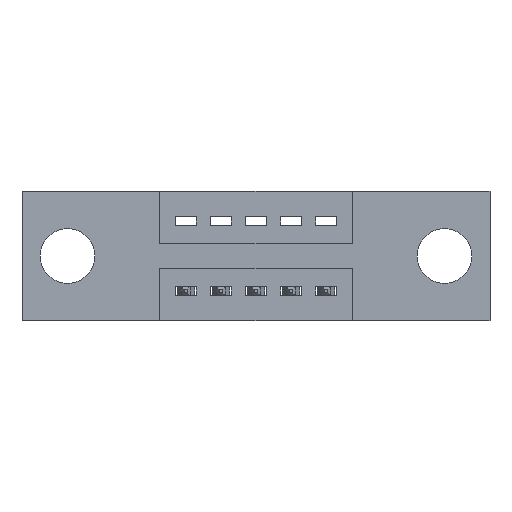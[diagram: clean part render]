
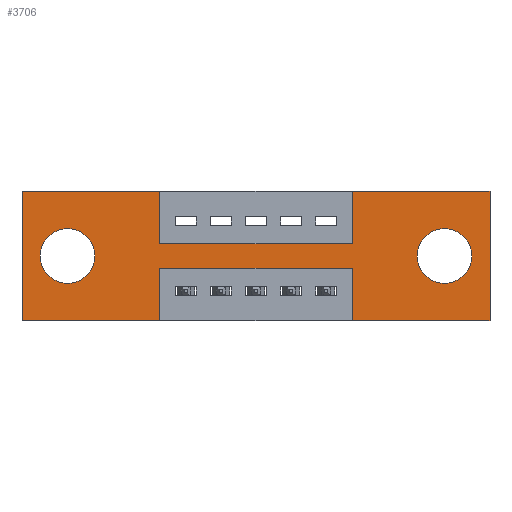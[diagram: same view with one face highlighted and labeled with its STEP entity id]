
A CAD part, front view. The second image highlights one B-rep face of the part: STEP entity #3706.
In plain terms, the highlighted planar face has unit normal (0, -1, 0).
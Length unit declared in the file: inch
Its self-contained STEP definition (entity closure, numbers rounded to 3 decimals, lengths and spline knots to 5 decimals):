
#21 = VERTEX_POINT ( 'NONE', #4066 ) ;
#74 = ORIENTED_EDGE ( 'NONE', *, *, #4020, .T. ) ;
#341 = CIRCLE ( 'NONE', #486, 0.078 ) ;
#416 = VERTEX_POINT ( 'NONE', #6061 ) ;
#418 = FACE_BOUND ( 'NONE', #1956, .T. ) ;
#486 = AXIS2_PLACEMENT_3D ( 'NONE', #2721, #8781, #7481 ) ;
#595 = AXIS2_PLACEMENT_3D ( 'NONE', #3343, #1869, #6625 ) ;
#641 = DIRECTION ( 'NONE',  ( 0., 1., 0. ) ) ;
#747 = AXIS2_PLACEMENT_3D ( 'NONE', #6677, #6643, #4599 ) ;
#905 = CARTESIAN_POINT ( 'NONE',  ( 0.9425, 0., -0.37 ) ) ;
#945 = VECTOR ( 'NONE', #3527, 39.37008 ) ;
#966 = VECTOR ( 'NONE', #6307, 39.37008 ) ;
#1000 = DIRECTION ( 'NONE',  ( 0., 0., 1. ) ) ;
#1029 = EDGE_CURVE ( 'NONE', #7774, #8764, #7888, .T. ) ;
#1031 = DIRECTION ( 'NONE',  ( 0., 0., -1. ) ) ;
#1033 = DIRECTION ( 'NONE',  ( -1., 0., 0. ) ) ;
#1087 = CARTESIAN_POINT ( 'NONE',  ( 1.335, 0., 0. ) ) ;
#1292 = LINE ( 'NONE', #8317, #966 ) ;
#1485 = EDGE_CURVE ( 'NONE', #3220, #4283, #3207, .T. ) ;
#1566 = CIRCLE ( 'NONE', #7570, 0.078 ) ;
#1573 = CARTESIAN_POINT ( 'NONE',  ( 1.205, 0., -0.107 ) ) ;
#1627 = ORIENTED_EDGE ( 'NONE', *, *, #7417, .T. ) ;
#1657 = CARTESIAN_POINT ( 'NONE',  ( 0.3925, 0., -0.15 ) ) ;
#1842 = DIRECTION ( 'NONE',  ( 1., 0., 0. ) ) ;
#1860 = ORIENTED_EDGE ( 'NONE', *, *, #8608, .F. ) ;
#1869 = DIRECTION ( 'NONE',  ( 0., -1., 0. ) ) ;
#1956 = EDGE_LOOP ( 'NONE', ( #74, #4392 ) ) ;
#2031 = CARTESIAN_POINT ( 'NONE',  ( 1.335, 0., 0. ) ) ;
#2058 = VERTEX_POINT ( 'NONE', #1657 ) ;
#2190 = LINE ( 'NONE', #3152, #5684 ) ;
#2250 = CARTESIAN_POINT ( 'NONE',  ( 0.3925, 0., -0.22 ) ) ;
#2300 = EDGE_CURVE ( 'NONE', #8406, #6482, #341, .T. ) ;
#2382 = VERTEX_POINT ( 'NONE', #8207 ) ;
#2653 = ORIENTED_EDGE ( 'NONE', *, *, #7358, .F. ) ;
#2720 = VERTEX_POINT ( 'NONE', #4637 ) ;
#2721 = CARTESIAN_POINT ( 'NONE',  ( 0.13, 0., -0.185 ) ) ;
#2741 = LINE ( 'NONE', #2250, #7955 ) ;
#2833 = EDGE_CURVE ( 'NONE', #6763, #5205, #5071, .T. ) ;
#2945 = ORIENTED_EDGE ( 'NONE', *, *, #3050, .F. ) ;
#3024 = VECTOR ( 'NONE', #6362, 39.37008 ) ;
#3050 = EDGE_CURVE ( 'NONE', #8764, #6763, #7743, .T. ) ;
#3066 = CARTESIAN_POINT ( 'NONE',  ( 0., 0., -0.37 ) ) ;
#3136 = VERTEX_POINT ( 'NONE', #3662 ) ;
#3152 = CARTESIAN_POINT ( 'NONE',  ( 0., 0., 0. ) ) ;
#3160 = DIRECTION ( 'NONE',  ( -1., 0., 0. ) ) ;
#3185 = DIRECTION ( 'NONE',  ( 0., 1., 0. ) ) ;
#3199 = LINE ( 'NONE', #7068, #7547 ) ;
#3207 = LINE ( 'NONE', #6512, #7558 ) ;
#3220 = VERTEX_POINT ( 'NONE', #905 ) ;
#3265 = EDGE_CURVE ( 'NONE', #4283, #2382, #2741, .T. ) ;
#3272 = FACE_BOUND ( 'NONE', #7664, .T. ) ;
#3328 = CARTESIAN_POINT ( 'NONE',  ( 0.9425, 0., 0. ) ) ;
#3343 = CARTESIAN_POINT ( 'NONE',  ( 0., 0., -0.37 ) ) ;
#3439 = CARTESIAN_POINT ( 'NONE',  ( 0.9425, 0., -0.22 ) ) ;
#3527 = DIRECTION ( 'NONE',  ( 1., 0., 0. ) ) ;
#3559 = CARTESIAN_POINT ( 'NONE',  ( 0.13, 0., -0.263 ) ) ;
#3580 = CARTESIAN_POINT ( 'NONE',  ( 0.3925, 0., -0.15 ) ) ;
#3662 = CARTESIAN_POINT ( 'NONE',  ( 1.205, 0., -0.263 ) ) ;
#3706 = ADVANCED_FACE ( 'NONE', ( #3272, #418, #6690 ), #3907, .T. ) ;
#3880 = DIRECTION ( 'NONE',  ( 0., 0., 1. ) ) ;
#3907 = PLANE ( 'NONE',  #595 ) ;
#3916 = CARTESIAN_POINT ( 'NONE',  ( 1.205, 0., -0.185 ) ) ;
#4020 = EDGE_CURVE ( 'NONE', #6482, #8406, #4306, .T. ) ;
#4048 = CIRCLE ( 'NONE', #747, 0.078 ) ;
#4066 = CARTESIAN_POINT ( 'NONE',  ( 0., 0., 0. ) ) ;
#4110 = VECTOR ( 'NONE', #7418, 39.37008 ) ;
#4111 = CARTESIAN_POINT ( 'NONE',  ( 0., 0., 0. ) ) ;
#4158 = ORIENTED_EDGE ( 'NONE', *, *, #3265, .F. ) ;
#4180 = EDGE_CURVE ( 'NONE', #7726, #3136, #1566, .T. ) ;
#4182 = LINE ( 'NONE', #5139, #6769 ) ;
#4283 = VERTEX_POINT ( 'NONE', #3439 ) ;
#4306 = CIRCLE ( 'NONE', #6682, 0.078 ) ;
#4392 = ORIENTED_EDGE ( 'NONE', *, *, #2300, .T. ) ;
#4572 = EDGE_LOOP ( 'NONE', ( #6908, #4158, #7731, #2653, #6101, #2945, #7096, #5273, #1860, #8136, #8319, #6239 ) ) ;
#4599 = DIRECTION ( 'NONE',  ( 0., 0., -1. ) ) ;
#4637 = CARTESIAN_POINT ( 'NONE',  ( 0.3925, 0., -0.37 ) ) ;
#4693 = EDGE_CURVE ( 'NONE', #21, #416, #2190, .T. ) ;
#4819 = LINE ( 'NONE', #3580, #3024 ) ;
#4924 = LINE ( 'NONE', #3066, #6543 ) ;
#5071 = LINE ( 'NONE', #2031, #4110 ) ;
#5094 = CARTESIAN_POINT ( 'NONE',  ( 0.13, 0., -0.185 ) ) ;
#5139 = CARTESIAN_POINT ( 'NONE',  ( 0.3925, 0., -0.37 ) ) ;
#5205 = VERTEX_POINT ( 'NONE', #5747 ) ;
#5273 = ORIENTED_EDGE ( 'NONE', *, *, #6084, .F. ) ;
#5286 = DIRECTION ( 'NONE',  ( 0., 0., -1. ) ) ;
#5455 = EDGE_CURVE ( 'NONE', #2382, #2720, #4182, .T. ) ;
#5545 = EDGE_CURVE ( 'NONE', #2720, #7024, #4924, .T. ) ;
#5552 = CARTESIAN_POINT ( 'NONE',  ( 0.13, 0., -0.107 ) ) ;
#5684 = VECTOR ( 'NONE', #1842, 39.37008 ) ;
#5747 = CARTESIAN_POINT ( 'NONE',  ( 1.335, 0., -0.37 ) ) ;
#5883 = DIRECTION ( 'NONE',  ( -1., 0., 0. ) ) ;
#5972 = VECTOR ( 'NONE', #3160, 39.37008 ) ;
#5986 = VECTOR ( 'NONE', #3880, 39.37008 ) ;
#6061 = CARTESIAN_POINT ( 'NONE',  ( 0.3925, 0., 0. ) ) ;
#6084 = EDGE_CURVE ( 'NONE', #2058, #7774, #4819, .T. ) ;
#6101 = ORIENTED_EDGE ( 'NONE', *, *, #2833, .F. ) ;
#6239 = ORIENTED_EDGE ( 'NONE', *, *, #5545, .F. ) ;
#6307 = DIRECTION ( 'NONE',  ( 0., 0., 1. ) ) ;
#6362 = DIRECTION ( 'NONE',  ( 1., 0., 0. ) ) ;
#6482 = VERTEX_POINT ( 'NONE', #5552 ) ;
#6499 = ORIENTED_EDGE ( 'NONE', *, *, #4180, .T. ) ;
#6512 = CARTESIAN_POINT ( 'NONE',  ( 0.9425, 0., -0.37 ) ) ;
#6543 = VECTOR ( 'NONE', #1033, 39.37008 ) ;
#6625 = DIRECTION ( 'NONE',  ( 0., 0., -1. ) ) ;
#6635 = CARTESIAN_POINT ( 'NONE',  ( 0.9425, 0., 0. ) ) ;
#6643 = DIRECTION ( 'NONE',  ( 0., 1., 0. ) ) ;
#6677 = CARTESIAN_POINT ( 'NONE',  ( 1.205, 0., -0.185 ) ) ;
#6682 = AXIS2_PLACEMENT_3D ( 'NONE', #5094, #3185, #7941 ) ;
#6690 = FACE_OUTER_BOUND ( 'NONE', #4572, .T. ) ;
#6763 = VERTEX_POINT ( 'NONE', #1087 ) ;
#6769 = VECTOR ( 'NONE', #7794, 39.37008 ) ;
#6908 = ORIENTED_EDGE ( 'NONE', *, *, #5455, .F. ) ;
#7024 = VERTEX_POINT ( 'NONE', #7852 ) ;
#7068 = CARTESIAN_POINT ( 'NONE',  ( 0.3925, 0., 0. ) ) ;
#7096 = ORIENTED_EDGE ( 'NONE', *, *, #1029, .F. ) ;
#7358 = EDGE_CURVE ( 'NONE', #5205, #3220, #7565, .T. ) ;
#7417 = EDGE_CURVE ( 'NONE', #3136, #7726, #4048, .T. ) ;
#7418 = DIRECTION ( 'NONE',  ( 0., 0., -1. ) ) ;
#7481 = DIRECTION ( 'NONE',  ( 0., 0., 1. ) ) ;
#7547 = VECTOR ( 'NONE', #1031, 39.37008 ) ;
#7558 = VECTOR ( 'NONE', #1000, 39.37008 ) ;
#7565 = LINE ( 'NONE', #7904, #5972 ) ;
#7570 = AXIS2_PLACEMENT_3D ( 'NONE', #3916, #641, #5286 ) ;
#7664 = EDGE_LOOP ( 'NONE', ( #6499, #1627 ) ) ;
#7726 = VERTEX_POINT ( 'NONE', #1573 ) ;
#7731 = ORIENTED_EDGE ( 'NONE', *, *, #1485, .F. ) ;
#7743 = LINE ( 'NONE', #4111, #945 ) ;
#7749 = CARTESIAN_POINT ( 'NONE',  ( 0.9425, 0., -0.15 ) ) ;
#7774 = VERTEX_POINT ( 'NONE', #7749 ) ;
#7794 = DIRECTION ( 'NONE',  ( 0., 0., -1. ) ) ;
#7852 = CARTESIAN_POINT ( 'NONE',  ( 0., 0., -0.37 ) ) ;
#7888 = LINE ( 'NONE', #6635, #5986 ) ;
#7904 = CARTESIAN_POINT ( 'NONE',  ( 0., 0., -0.37 ) ) ;
#7941 = DIRECTION ( 'NONE',  ( 0., 0., 1. ) ) ;
#7955 = VECTOR ( 'NONE', #5883, 39.37008 ) ;
#8136 = ORIENTED_EDGE ( 'NONE', *, *, #4693, .F. ) ;
#8207 = CARTESIAN_POINT ( 'NONE',  ( 0.3925, 0., -0.22 ) ) ;
#8317 = CARTESIAN_POINT ( 'NONE',  ( 0., 0., 0. ) ) ;
#8319 = ORIENTED_EDGE ( 'NONE', *, *, #8387, .F. ) ;
#8387 = EDGE_CURVE ( 'NONE', #7024, #21, #1292, .T. ) ;
#8406 = VERTEX_POINT ( 'NONE', #3559 ) ;
#8608 = EDGE_CURVE ( 'NONE', #416, #2058, #3199, .T. ) ;
#8764 = VERTEX_POINT ( 'NONE', #3328 ) ;
#8781 = DIRECTION ( 'NONE',  ( 0., 1., 0. ) ) ;
